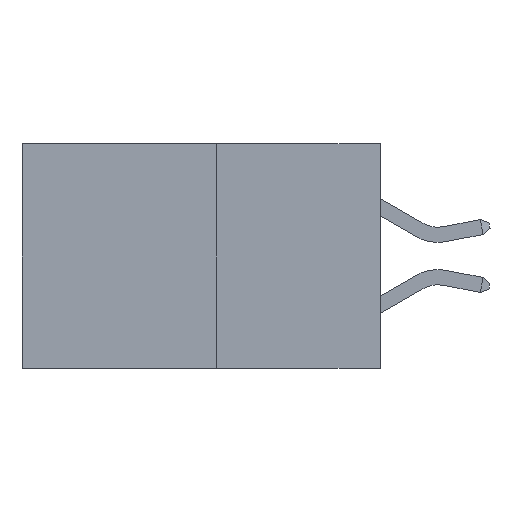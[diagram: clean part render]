
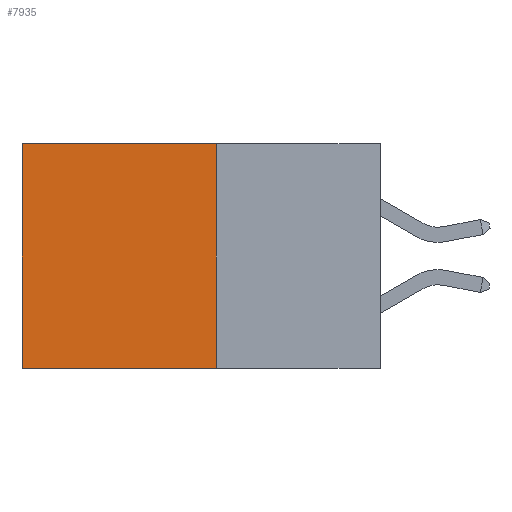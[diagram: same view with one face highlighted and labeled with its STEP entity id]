
A CAD part, left-side view. The second image highlights one B-rep face of the part: STEP entity #7935.
In plain terms, the highlighted planar face has unit normal (-1, 0, 0).
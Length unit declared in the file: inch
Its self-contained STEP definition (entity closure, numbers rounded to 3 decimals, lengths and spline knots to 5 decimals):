
#85 = VERTEX_POINT ( 'NONE', #13295 ) ;
#143 = DIRECTION ( 'NONE',  ( 1., 0., 0. ) ) ;
#513 = VECTOR ( 'NONE', #18826, 39.37008 ) ;
#1161 = LINE ( 'NONE', #7295, #513 ) ;
#1503 = ORIENTED_EDGE ( 'NONE', *, *, #16626, .F. ) ;
#1670 = LINE ( 'NONE', #8165, #21155 ) ;
#1946 = CARTESIAN_POINT ( 'NONE',  ( 0.277, 0.59, -0.37 ) ) ;
#1991 = FACE_OUTER_BOUND ( 'NONE', #4819, .T. ) ;
#4819 = EDGE_LOOP ( 'NONE', ( #12343, #13781, #1503, #12475 ) ) ;
#5953 = DIRECTION ( 'NONE',  ( 0., 1., 0. ) ) ;
#7295 = CARTESIAN_POINT ( 'NONE',  ( 0.277, 0.27, -0.37 ) ) ;
#7776 = CARTESIAN_POINT ( 'NONE',  ( 0.277, 0.27, 0. ) ) ;
#7935 = ADVANCED_FACE ( 'NONE', ( #1991 ), #12071, .F. ) ;
#8165 = CARTESIAN_POINT ( 'NONE',  ( 0.277, 0.59, -0.37 ) ) ;
#8169 = AXIS2_PLACEMENT_3D ( 'NONE', #21550, #143, #14003 ) ;
#9752 = LINE ( 'NONE', #15677, #14273 ) ;
#9814 = VERTEX_POINT ( 'NONE', #1946 ) ;
#10600 = VERTEX_POINT ( 'NONE', #14362 ) ;
#10791 = EDGE_CURVE ( 'NONE', #23380, #85, #15407, .T. ) ;
#12071 = PLANE ( 'NONE',  #8169 ) ;
#12343 = ORIENTED_EDGE ( 'NONE', *, *, #24219, .T. ) ;
#12475 = ORIENTED_EDGE ( 'NONE', *, *, #10791, .T. ) ;
#13295 = CARTESIAN_POINT ( 'NONE',  ( 0.277, 0.59, 0. ) ) ;
#13781 = ORIENTED_EDGE ( 'NONE', *, *, #24686, .F. ) ;
#14003 = DIRECTION ( 'NONE',  ( 0., 0., -1. ) ) ;
#14273 = VECTOR ( 'NONE', #5953, 39.37008 ) ;
#14362 = CARTESIAN_POINT ( 'NONE',  ( 0.277, 0.27, -0.37 ) ) ;
#15407 = LINE ( 'NONE', #18668, #19839 ) ;
#15677 = CARTESIAN_POINT ( 'NONE',  ( 0.277, 0.27, -0.37 ) ) ;
#16626 = EDGE_CURVE ( 'NONE', #23380, #10600, #1161, .T. ) ;
#18668 = CARTESIAN_POINT ( 'NONE',  ( 0.277, 0.27, 0. ) ) ;
#18826 = DIRECTION ( 'NONE',  ( 0., 0., -1. ) ) ;
#19657 = DIRECTION ( 'NONE',  ( 0., 0., -1. ) ) ;
#19839 = VECTOR ( 'NONE', #20599, 39.37008 ) ;
#20599 = DIRECTION ( 'NONE',  ( 0., 1., 0. ) ) ;
#21155 = VECTOR ( 'NONE', #19657, 39.37008 ) ;
#21550 = CARTESIAN_POINT ( 'NONE',  ( 0.277, 0.27, -0.37 ) ) ;
#23380 = VERTEX_POINT ( 'NONE', #7776 ) ;
#24219 = EDGE_CURVE ( 'NONE', #85, #9814, #1670, .T. ) ;
#24686 = EDGE_CURVE ( 'NONE', #10600, #9814, #9752, .T. ) ;
